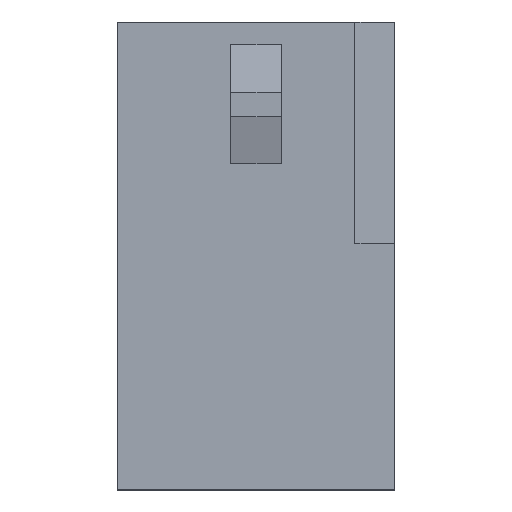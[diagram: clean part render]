
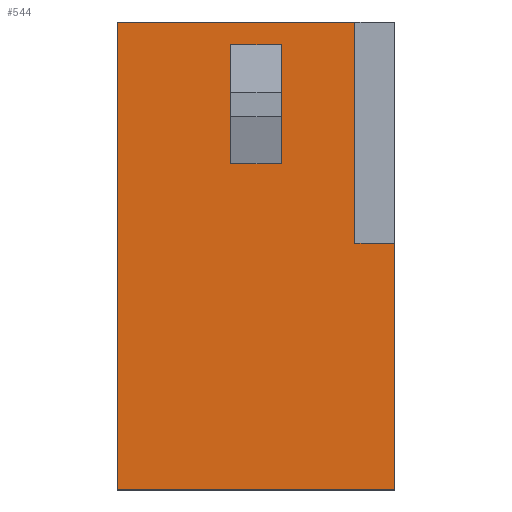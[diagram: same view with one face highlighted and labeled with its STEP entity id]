
A CAD part, top view. The second image highlights one B-rep face of the part: STEP entity #544.
In plain terms, the highlighted planar face has unit normal (0, 0, 1).
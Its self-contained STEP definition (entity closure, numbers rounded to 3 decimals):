
#19 = ORIENTED_EDGE ( 'NONE', *, *, #106, .F. ) ;
#46 = VERTEX_POINT ( 'NONE', #1210 ) ;
#64 = CARTESIAN_POINT ( 'NONE',  ( 10.249, -11.176, 2.54 ) ) ;
#65 = CARTESIAN_POINT ( 'NONE',  ( 8.445, 44.802, 2.54 ) ) ;
#84 = ORIENTED_EDGE ( 'NONE', *, *, #612, .T. ) ;
#106 = EDGE_CURVE ( 'NONE', #46, #1614, #1884, .T. ) ;
#238 = AXIS2_PLACEMENT_3D ( 'NONE', #1196, #916, #398 ) ;
#280 = VECTOR ( 'NONE', #1699, 1000. ) ;
#286 = VECTOR ( 'NONE', #3083, 1000. ) ;
#288 = CARTESIAN_POINT ( 'NONE',  ( -2.324, 0., 2.54 ) ) ;
#339 = DIRECTION ( 'NONE',  ( 0., 1., 0. ) ) ;
#394 = CARTESIAN_POINT ( 'NONE',  ( -2.324, -11.176, 2.54 ) ) ;
#398 = DIRECTION ( 'NONE',  ( 1., 0., 0. ) ) ;
#412 = DIRECTION ( 'NONE',  ( 0., -1., 0. ) ) ;
#452 = CARTESIAN_POINT ( 'NONE',  ( -2.324, 10.033, 2.54 ) ) ;
#489 = VECTOR ( 'NONE', #339, 1000. ) ;
#540 = DIRECTION ( 'NONE',  ( 0., -1., 0. ) ) ;
#544 = ADVANCED_FACE ( 'NONE', ( #1561, #2869 ), #3018, .T. ) ;
#612 = EDGE_CURVE ( 'NONE', #2699, #750, #1759, .T. ) ;
#681 = EDGE_LOOP ( 'NONE', ( #951, #2933, #915, #2832, #84, #1473 ) ) ;
#715 = CARTESIAN_POINT ( 'NONE',  ( 7.339, 8.991, 2.54 ) ) ;
#725 = EDGE_CURVE ( 'NONE', #2699, #1014, #1169, .T. ) ;
#740 = LINE ( 'NONE', #452, #1182 ) ;
#750 = VERTEX_POINT ( 'NONE', #2797 ) ;
#778 = LINE ( 'NONE', #1868, #1101 ) ;
#799 = CARTESIAN_POINT ( 'NONE',  ( 8.445, 10.033, 2.54 ) ) ;
#915 = ORIENTED_EDGE ( 'NONE', *, *, #1035, .F. ) ;
#916 = DIRECTION ( 'NONE',  ( 0., 0., 1. ) ) ;
#951 = ORIENTED_EDGE ( 'NONE', *, *, #1616, .F. ) ;
#968 = VECTOR ( 'NONE', #1230, 1000. ) ;
#986 = CARTESIAN_POINT ( 'NONE',  ( -2.324, -11.176, 2.54 ) ) ;
#990 = VERTEX_POINT ( 'NONE', #3338 ) ;
#1014 = VERTEX_POINT ( 'NONE', #2803 ) ;
#1035 = EDGE_CURVE ( 'NONE', #1014, #2219, #740, .T. ) ;
#1039 = DIRECTION ( 'NONE',  ( 0., 1., 0. ) ) ;
#1044 = VECTOR ( 'NONE', #412, 1000. ) ;
#1101 = VECTOR ( 'NONE', #540, 1000. ) ;
#1159 = CARTESIAN_POINT ( 'NONE',  ( -2.324, -11.176, 2.54 ) ) ;
#1169 = LINE ( 'NONE', #986, #968 ) ;
#1175 = CARTESIAN_POINT ( 'NONE',  ( 8.445, 0., 2.54 ) ) ;
#1182 = VECTOR ( 'NONE', #2518, 1000. ) ;
#1196 = CARTESIAN_POINT ( 'NONE',  ( -2.324, -11.176, 2.54 ) ) ;
#1210 = CARTESIAN_POINT ( 'NONE',  ( 5.105, 8.991, 2.54 ) ) ;
#1230 = DIRECTION ( 'NONE',  ( 0., 1., 0. ) ) ;
#1285 = EDGE_CURVE ( 'NONE', #1614, #2734, #778, .T. ) ;
#1305 = VECTOR ( 'NONE', #2881, 1000. ) ;
#1325 = EDGE_CURVE ( 'NONE', #750, #3088, #2910, .T. ) ;
#1358 = ORIENTED_EDGE ( 'NONE', *, *, #1285, .F. ) ;
#1473 = ORIENTED_EDGE ( 'NONE', *, *, #1325, .T. ) ;
#1561 = FACE_BOUND ( 'NONE', #2621, .T. ) ;
#1614 = VERTEX_POINT ( 'NONE', #3402 ) ;
#1616 = EDGE_CURVE ( 'NONE', #2019, #3088, #2529, .T. ) ;
#1699 = DIRECTION ( 'NONE',  ( -1., 0., 0. ) ) ;
#1759 = LINE ( 'NONE', #394, #2541 ) ;
#1815 = CARTESIAN_POINT ( 'NONE',  ( 5.105, 8.992, 2.54 ) ) ;
#1868 = CARTESIAN_POINT ( 'NONE',  ( 2.819, 8.992, 2.54 ) ) ;
#1872 = LINE ( 'NONE', #1815, #2362 ) ;
#1884 = LINE ( 'NONE', #715, #286 ) ;
#1976 = CARTESIAN_POINT ( 'NONE',  ( 2.819, 3.608, 2.54 ) ) ;
#2019 = VERTEX_POINT ( 'NONE', #1175 ) ;
#2219 = VERTEX_POINT ( 'NONE', #799 ) ;
#2229 = LINE ( 'NONE', #2989, #280 ) ;
#2338 = ORIENTED_EDGE ( 'NONE', *, *, #3084, .F. ) ;
#2362 = VECTOR ( 'NONE', #1039, 1000. ) ;
#2442 = LINE ( 'NONE', #65, #1044 ) ;
#2518 = DIRECTION ( 'NONE',  ( 1., 0., 0. ) ) ;
#2529 = LINE ( 'NONE', #288, #1305 ) ;
#2541 = VECTOR ( 'NONE', #3291, 1000. ) ;
#2609 = CARTESIAN_POINT ( 'NONE',  ( 10.249, 0., 2.54 ) ) ;
#2621 = EDGE_LOOP ( 'NONE', ( #2653, #1358, #19, #2338 ) ) ;
#2653 = ORIENTED_EDGE ( 'NONE', *, *, #2810, .T. ) ;
#2699 = VERTEX_POINT ( 'NONE', #1159 ) ;
#2734 = VERTEX_POINT ( 'NONE', #1976 ) ;
#2797 = CARTESIAN_POINT ( 'NONE',  ( 10.249, -11.176, 2.54 ) ) ;
#2803 = CARTESIAN_POINT ( 'NONE',  ( -2.324, 10.033, 2.54 ) ) ;
#2810 = EDGE_CURVE ( 'NONE', #990, #2734, #2229, .T. ) ;
#2832 = ORIENTED_EDGE ( 'NONE', *, *, #725, .F. ) ;
#2869 = FACE_OUTER_BOUND ( 'NONE', #681, .T. ) ;
#2881 = DIRECTION ( 'NONE',  ( 1., 0., 0. ) ) ;
#2910 = LINE ( 'NONE', #64, #489 ) ;
#2933 = ORIENTED_EDGE ( 'NONE', *, *, #3328, .F. ) ;
#2989 = CARTESIAN_POINT ( 'NONE',  ( 7.339, 3.608, 2.54 ) ) ;
#3018 = PLANE ( 'NONE',  #238 ) ;
#3083 = DIRECTION ( 'NONE',  ( -1., 0., 0. ) ) ;
#3084 = EDGE_CURVE ( 'NONE', #990, #46, #1872, .T. ) ;
#3088 = VERTEX_POINT ( 'NONE', #2609 ) ;
#3291 = DIRECTION ( 'NONE',  ( 1., 0., 0. ) ) ;
#3328 = EDGE_CURVE ( 'NONE', #2219, #2019, #2442, .T. ) ;
#3338 = CARTESIAN_POINT ( 'NONE',  ( 5.105, 3.608, 2.54 ) ) ;
#3402 = CARTESIAN_POINT ( 'NONE',  ( 2.819, 8.991, 2.54 ) ) ;
